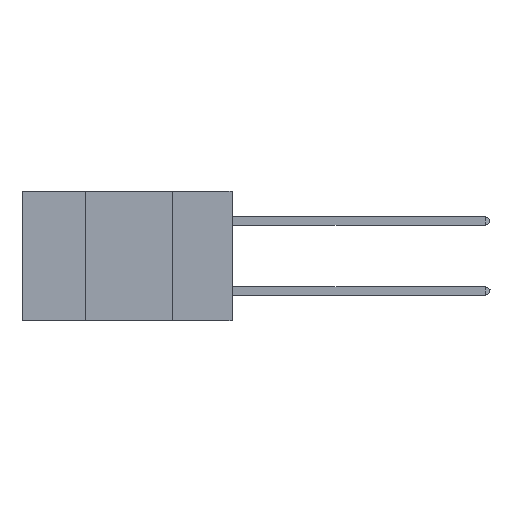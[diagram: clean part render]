
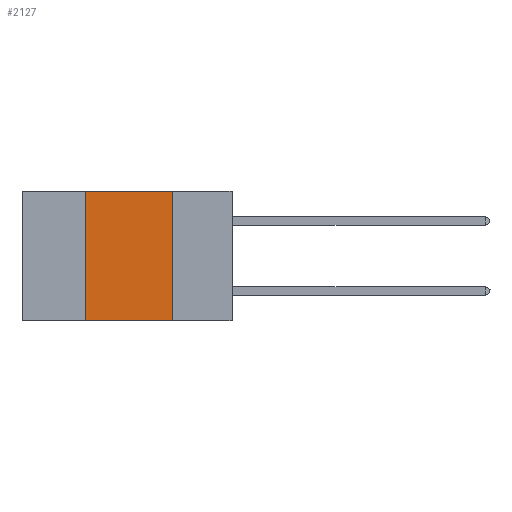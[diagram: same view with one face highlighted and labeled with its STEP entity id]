
A CAD part, left-side view. The second image highlights one B-rep face of the part: STEP entity #2127.
In plain terms, the highlighted planar face has unit normal (-1, 0, 0).
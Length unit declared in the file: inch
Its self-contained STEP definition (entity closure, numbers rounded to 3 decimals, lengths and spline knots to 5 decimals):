
#1232 = CARTESIAN_POINT ( 'NONE',  ( 0., 0.6, 0. ) ) ;
#1483 = LINE ( 'NONE', #17964, #13022 ) ;
#2127 = ADVANCED_FACE ( 'NONE', ( #10123 ), #10372, .F. ) ;
#3140 = VECTOR ( 'NONE', #19626, 39.37008 ) ;
#3212 = VECTOR ( 'NONE', #10047, 39.37008 ) ;
#3857 = EDGE_CURVE ( 'NONE', #6560, #7090, #6874, .T. ) ;
#4626 = CARTESIAN_POINT ( 'NONE',  ( 0., 0.42, -0.37 ) ) ;
#4862 = DIRECTION ( 'NONE',  ( 1., 0., 0. ) ) ;
#5403 = ORIENTED_EDGE ( 'NONE', *, *, #7617, .F. ) ;
#6560 = VERTEX_POINT ( 'NONE', #13465 ) ;
#6706 = DIRECTION ( 'NONE',  ( 0., 0., -1. ) ) ;
#6874 = LINE ( 'NONE', #15746, #3140 ) ;
#7090 = VERTEX_POINT ( 'NONE', #11903 ) ;
#7617 = EDGE_CURVE ( 'NONE', #10018, #6560, #8122, .T. ) ;
#8122 = LINE ( 'NONE', #18181, #3212 ) ;
#10018 = VERTEX_POINT ( 'NONE', #13324 ) ;
#10047 = DIRECTION ( 'NONE',  ( 0., -1., 0. ) ) ;
#10123 = FACE_OUTER_BOUND ( 'NONE', #11028, .T. ) ;
#10372 = PLANE ( 'NONE',  #11804 ) ;
#10519 = CARTESIAN_POINT ( 'NONE',  ( 0., 0.6, -0.37 ) ) ;
#10602 = DIRECTION ( 'NONE',  ( 0., -1., 0. ) ) ;
#11028 = EDGE_LOOP ( 'NONE', ( #16470, #5403, #16796, #17592 ) ) ;
#11599 = EDGE_CURVE ( 'NONE', #18396, #7090, #19439, .T. ) ;
#11804 = AXIS2_PLACEMENT_3D ( 'NONE', #1232, #4862, #6706 ) ;
#11903 = CARTESIAN_POINT ( 'NONE',  ( 0., 0.17, -0.37 ) ) ;
#12490 = DIRECTION ( 'NONE',  ( 0., 0., 1. ) ) ;
#13022 = VECTOR ( 'NONE', #12490, 39.37008 ) ;
#13324 = CARTESIAN_POINT ( 'NONE',  ( 0., 0.42, 0. ) ) ;
#13465 = CARTESIAN_POINT ( 'NONE',  ( 0., 0.17, 0. ) ) ;
#15746 = CARTESIAN_POINT ( 'NONE',  ( 0., 0.17, 0. ) ) ;
#16470 = ORIENTED_EDGE ( 'NONE', *, *, #3857, .F. ) ;
#16796 = ORIENTED_EDGE ( 'NONE', *, *, #23558, .F. ) ;
#17592 = ORIENTED_EDGE ( 'NONE', *, *, #11599, .T. ) ;
#17964 = CARTESIAN_POINT ( 'NONE',  ( 0., 0.42, 0. ) ) ;
#18181 = CARTESIAN_POINT ( 'NONE',  ( 0., 0.6, 0. ) ) ;
#18396 = VERTEX_POINT ( 'NONE', #4626 ) ;
#19439 = LINE ( 'NONE', #10519, #20280 ) ;
#19626 = DIRECTION ( 'NONE',  ( 0., 0., -1. ) ) ;
#20280 = VECTOR ( 'NONE', #10602, 39.37008 ) ;
#23558 = EDGE_CURVE ( 'NONE', #18396, #10018, #1483, .T. ) ;
